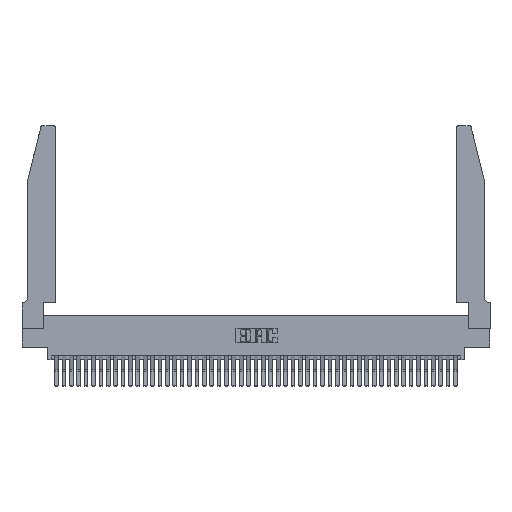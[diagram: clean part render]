
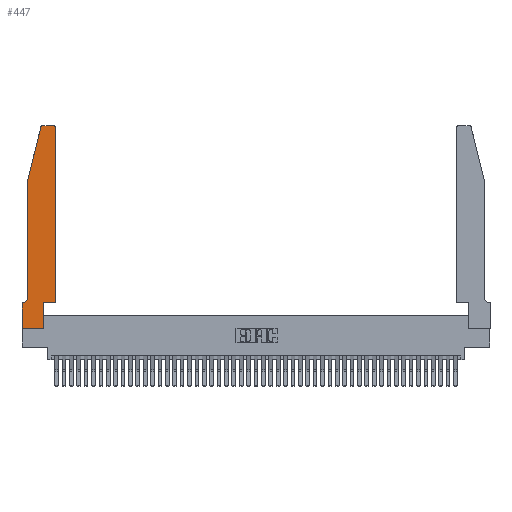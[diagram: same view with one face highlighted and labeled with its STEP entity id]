
A CAD part, top view. The second image highlights one B-rep face of the part: STEP entity #447.
In plain terms, the highlighted planar face has unit normal (0, 0, 1).
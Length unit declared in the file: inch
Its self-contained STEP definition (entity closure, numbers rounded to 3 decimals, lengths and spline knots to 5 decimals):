
#447 = ADVANCED_FACE ( 'NONE', ( #30913 ), #37221, .T. ) ;
#463 = LINE ( 'NONE', #20594, #21248 ) ;
#1163 = CARTESIAN_POINT ( 'NONE',  ( 0.0755, 2., 0.37 ) ) ;
#1435 = ORIENTED_EDGE ( 'NONE', *, *, #6084, .T. ) ;
#1758 = DIRECTION ( 'NONE',  ( -1., 0., 0. ) ) ;
#1837 = CARTESIAN_POINT ( 'NONE',  ( 0.2865, 0.35, 0.37 ) ) ;
#2335 = EDGE_CURVE ( 'NONE', #25333, #40328, #34635, .T. ) ;
#2625 = CARTESIAN_POINT ( 'NONE',  ( 0., 0.35, 0.37 ) ) ;
#3387 = LINE ( 'NONE', #9827, #34214 ) ;
#3791 = ORIENTED_EDGE ( 'NONE', *, *, #4423, .T. ) ;
#4197 = VERTEX_POINT ( 'NONE', #15764 ) ;
#4423 = EDGE_CURVE ( 'NONE', #8046, #30609, #31054, .T. ) ;
#5084 = EDGE_CURVE ( 'NONE', #4197, #8046, #34949, .T. ) ;
#5197 = CARTESIAN_POINT ( 'NONE',  ( 0.2865, 0.35, 0.37 ) ) ;
#5504 = EDGE_CURVE ( 'NONE', #27647, #24235, #22586, .T. ) ;
#6084 = EDGE_CURVE ( 'NONE', #23175, #21379, #463, .T. ) ;
#6901 = CARTESIAN_POINT ( 'NONE',  ( 0.4505, 2.72, 0.37 ) ) ;
#6927 = ORIENTED_EDGE ( 'NONE', *, *, #11557, .T. ) ;
#7263 = CARTESIAN_POINT ( 'NONE',  ( 0.284, 2.75, 0.37 ) ) ;
#7716 = DIRECTION ( 'NONE',  ( 0., -1., 0. ) ) ;
#7744 = VECTOR ( 'NONE', #7716, 39.37008 ) ;
#8046 = VERTEX_POINT ( 'NONE', #5197 ) ;
#8805 = CARTESIAN_POINT ( 'NONE',  ( 0., 0.35, 0.37 ) ) ;
#9351 = VERTEX_POINT ( 'NONE', #7263 ) ;
#9486 = DIRECTION ( 'NONE',  ( 0., 0., 1. ) ) ;
#9827 = CARTESIAN_POINT ( 'NONE',  ( 0.2605, 2.75, 0.37 ) ) ;
#9957 = AXIS2_PLACEMENT_3D ( 'NONE', #40734, #19289, #1758 ) ;
#10322 = EDGE_LOOP ( 'NONE', ( #32216, #37114, #38824, #34930, #15198, #27966, #1435, #6927, #41491, #3791, #16183, #11367 ) ) ;
#11367 = ORIENTED_EDGE ( 'NONE', *, *, #2335, .T. ) ;
#11557 = EDGE_CURVE ( 'NONE', #21379, #4197, #17015, .T. ) ;
#12225 = EDGE_CURVE ( 'NONE', #9351, #27647, #36042, .T. ) ;
#12288 = DIRECTION ( 'NONE',  ( -0.239, -0.971, 0. ) ) ;
#12418 = EDGE_CURVE ( 'NONE', #30609, #25333, #33812, .T. ) ;
#13277 = EDGE_CURVE ( 'NONE', #24235, #23796, #33526, .T. ) ;
#13664 = VECTOR ( 'NONE', #22610, 39.37008 ) ;
#15198 = ORIENTED_EDGE ( 'NONE', *, *, #43077, .T. ) ;
#15764 = CARTESIAN_POINT ( 'NONE',  ( 0.2865, 0., 0.37 ) ) ;
#16183 = ORIENTED_EDGE ( 'NONE', *, *, #12418, .T. ) ;
#16266 = CARTESIAN_POINT ( 'NONE',  ( 0.4505, 0.35, 0.37 ) ) ;
#17015 = LINE ( 'NONE', #38975, #26514 ) ;
#17454 = AXIS2_PLACEMENT_3D ( 'NONE', #24592, #25661, #32402 ) ;
#18150 = CIRCLE ( 'NONE', #9957, 0.07 ) ;
#18851 = AXIS2_PLACEMENT_3D ( 'NONE', #2625, #9486, #20615 ) ;
#19289 = DIRECTION ( 'NONE',  ( 0., 0., -1. ) ) ;
#20594 = CARTESIAN_POINT ( 'NONE',  ( 0., 0., 0.37 ) ) ;
#20615 = DIRECTION ( 'NONE',  ( 1., 0., 0. ) ) ;
#21248 = VECTOR ( 'NONE', #42164, 39.37008 ) ;
#21379 = VERTEX_POINT ( 'NONE', #37536 ) ;
#21731 = LINE ( 'NONE', #31348, #39131 ) ;
#22331 = DIRECTION ( 'NONE',  ( 0., 0., 1. ) ) ;
#22451 = CARTESIAN_POINT ( 'NONE',  ( 0.4505, 0.35, 0.37 ) ) ;
#22586 = LINE ( 'NONE', #33570, #30483 ) ;
#22610 = DIRECTION ( 'NONE',  ( 0., 1., 0. ) ) ;
#23175 = VERTEX_POINT ( 'NONE', #8805 ) ;
#23796 = VERTEX_POINT ( 'NONE', #41783 ) ;
#24235 = VERTEX_POINT ( 'NONE', #32854 ) ;
#24592 = CARTESIAN_POINT ( 'NONE',  ( 0.4205, 2.72, 0.37 ) ) ;
#25333 = VERTEX_POINT ( 'NONE', #6901 ) ;
#25661 = DIRECTION ( 'NONE',  ( 0., 0., 1. ) ) ;
#26112 = DIRECTION ( 'NONE',  ( 1., 0., 0. ) ) ;
#26514 = VECTOR ( 'NONE', #32101, 39.37008 ) ;
#27647 = VERTEX_POINT ( 'NONE', #33054 ) ;
#27874 = DIRECTION ( 'NONE',  ( -1., 0., 0. ) ) ;
#27966 = ORIENTED_EDGE ( 'NONE', *, *, #35180, .T. ) ;
#28287 = VECTOR ( 'NONE', #41088, 39.37008 ) ;
#30483 = VECTOR ( 'NONE', #12288, 39.37008 ) ;
#30609 = VERTEX_POINT ( 'NONE', #16266 ) ;
#30913 = FACE_OUTER_BOUND ( 'NONE', #10322, .T. ) ;
#31054 = LINE ( 'NONE', #22451, #28287 ) ;
#31348 = CARTESIAN_POINT ( 'NONE',  ( 0.0755, 0.35, 0.37 ) ) ;
#32101 = DIRECTION ( 'NONE',  ( 1., 0., 0. ) ) ;
#32216 = ORIENTED_EDGE ( 'NONE', *, *, #34005, .T. ) ;
#32402 = DIRECTION ( 'NONE',  ( 1., 0., 0. ) ) ;
#32676 = VECTOR ( 'NONE', #44051, 39.37008 ) ;
#32854 = CARTESIAN_POINT ( 'NONE',  ( 0.0755, 2., 0.37 ) ) ;
#33054 = CARTESIAN_POINT ( 'NONE',  ( 0.25487, 2.72718, 0.37 ) ) ;
#33526 = LINE ( 'NONE', #1163, #7744 ) ;
#33570 = CARTESIAN_POINT ( 'NONE',  ( 0.0755, 2., 0.37 ) ) ;
#33812 = LINE ( 'NONE', #44208, #32676 ) ;
#34005 = EDGE_CURVE ( 'NONE', #40328, #9351, #3387, .T. ) ;
#34214 = VECTOR ( 'NONE', #27874, 39.37008 ) ;
#34635 = CIRCLE ( 'NONE', #17454, 0.03 ) ;
#34930 = ORIENTED_EDGE ( 'NONE', *, *, #13277, .T. ) ;
#34949 = LINE ( 'NONE', #1837, #13664 ) ;
#35180 = EDGE_CURVE ( 'NONE', #38977, #23175, #21731, .T. ) ;
#36042 = CIRCLE ( 'NONE', #40440, 0.03 ) ;
#36759 = CARTESIAN_POINT ( 'NONE',  ( 0.284, 2.72, 0.37 ) ) ;
#37114 = ORIENTED_EDGE ( 'NONE', *, *, #12225, .T. ) ;
#37221 = PLANE ( 'NONE',  #18851 ) ;
#37536 = CARTESIAN_POINT ( 'NONE',  ( 0., 0., 0.37 ) ) ;
#38824 = ORIENTED_EDGE ( 'NONE', *, *, #5504, .T. ) ;
#38975 = CARTESIAN_POINT ( 'NONE',  ( 0., 0., 0.37 ) ) ;
#38977 = VERTEX_POINT ( 'NONE', #39523 ) ;
#39131 = VECTOR ( 'NONE', #45309, 39.37008 ) ;
#39523 = CARTESIAN_POINT ( 'NONE',  ( 0.0055, 0.35, 0.37 ) ) ;
#40328 = VERTEX_POINT ( 'NONE', #42166 ) ;
#40440 = AXIS2_PLACEMENT_3D ( 'NONE', #36759, #22331, #26112 ) ;
#40734 = CARTESIAN_POINT ( 'NONE',  ( 0.0055, 0.42, 0.37 ) ) ;
#41088 = DIRECTION ( 'NONE',  ( 1., 0., 0. ) ) ;
#41491 = ORIENTED_EDGE ( 'NONE', *, *, #5084, .T. ) ;
#41783 = CARTESIAN_POINT ( 'NONE',  ( 0.0755, 0.42, 0.37 ) ) ;
#42164 = DIRECTION ( 'NONE',  ( 0., -1., 0. ) ) ;
#42166 = CARTESIAN_POINT ( 'NONE',  ( 0.4205, 2.75, 0.37 ) ) ;
#43077 = EDGE_CURVE ( 'NONE', #23796, #38977, #18150, .T. ) ;
#44051 = DIRECTION ( 'NONE',  ( 0., 1., 0. ) ) ;
#44208 = CARTESIAN_POINT ( 'NONE',  ( 0.4505, 0.35, 0.37 ) ) ;
#45309 = DIRECTION ( 'NONE',  ( -1., 0., 0. ) ) ;
